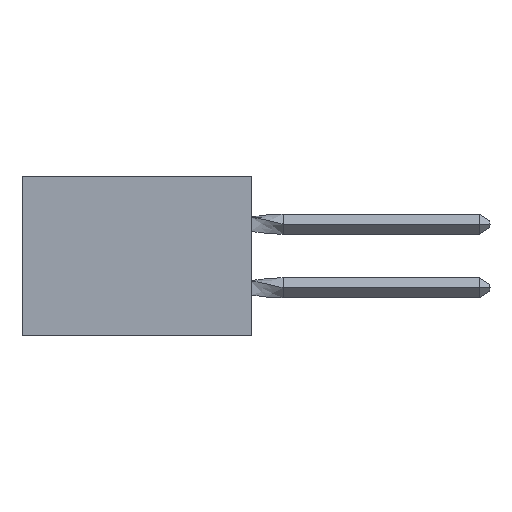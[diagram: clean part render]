
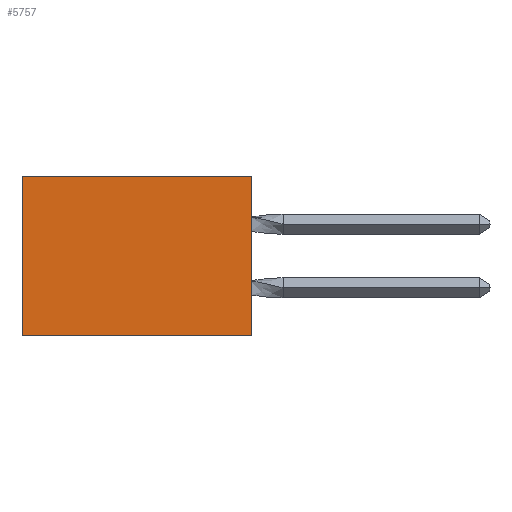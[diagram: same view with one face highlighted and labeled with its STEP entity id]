
A CAD part, left-side view. The second image highlights one B-rep face of the part: STEP entity #5757.
In plain terms, the highlighted planar face has unit normal (-1, 0, 0).
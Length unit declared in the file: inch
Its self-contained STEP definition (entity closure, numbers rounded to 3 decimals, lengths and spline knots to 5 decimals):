
#210 = EDGE_LOOP ( 'NONE', ( #7319, #8463, #7004, #6619 ) ) ;
#682 = VERTEX_POINT ( 'NONE', #9367 ) ;
#1037 = DIRECTION ( 'NONE',  ( 0., 0., -1. ) ) ;
#1528 = CARTESIAN_POINT ( 'NONE',  ( 0.305, 0.72, 0. ) ) ;
#1674 = DIRECTION ( 'NONE',  ( 0., 0., -1. ) ) ;
#1852 = EDGE_CURVE ( 'NONE', #682, #4171, #11782, .T. ) ;
#2416 = EDGE_CURVE ( 'NONE', #11622, #5801, #9221, .T. ) ;
#3059 = DIRECTION ( 'NONE',  ( 0., 1., 0. ) ) ;
#3100 = CARTESIAN_POINT ( 'NONE',  ( 0.305, 0., -0.5 ) ) ;
#3470 = AXIS2_PLACEMENT_3D ( 'NONE', #13197, #12264, #11199 ) ;
#3855 = VECTOR ( 'NONE', #3059, 39.37008 ) ;
#4153 = CARTESIAN_POINT ( 'NONE',  ( 0.305, 0.72, -0.5 ) ) ;
#4171 = VERTEX_POINT ( 'NONE', #1528 ) ;
#4537 = VECTOR ( 'NONE', #1037, 39.37008 ) ;
#5192 = LINE ( 'NONE', #12536, #4537 ) ;
#5757 = ADVANCED_FACE ( 'NONE', ( #7656 ), #6988, .F. ) ;
#5801 = VERTEX_POINT ( 'NONE', #4153 ) ;
#6090 = DIRECTION ( 'NONE',  ( 0., 1., 0. ) ) ;
#6619 = ORIENTED_EDGE ( 'NONE', *, *, #1852, .T. ) ;
#6805 = VECTOR ( 'NONE', #1674, 39.37008 ) ;
#6988 = PLANE ( 'NONE',  #3470 ) ;
#7004 = ORIENTED_EDGE ( 'NONE', *, *, #11348, .F. ) ;
#7319 = ORIENTED_EDGE ( 'NONE', *, *, #13141, .T. ) ;
#7656 = FACE_OUTER_BOUND ( 'NONE', #210, .T. ) ;
#8463 = ORIENTED_EDGE ( 'NONE', *, *, #2416, .F. ) ;
#8894 = CARTESIAN_POINT ( 'NONE',  ( 0.305, 0., -0.5 ) ) ;
#9221 = LINE ( 'NONE', #3100, #9873 ) ;
#9367 = CARTESIAN_POINT ( 'NONE',  ( 0.305, 0., 0. ) ) ;
#9584 = LINE ( 'NONE', #13282, #6805 ) ;
#9873 = VECTOR ( 'NONE', #6090, 39.37008 ) ;
#11199 = DIRECTION ( 'NONE',  ( 0., 0., -1. ) ) ;
#11348 = EDGE_CURVE ( 'NONE', #682, #11622, #5192, .T. ) ;
#11622 = VERTEX_POINT ( 'NONE', #8894 ) ;
#11782 = LINE ( 'NONE', #13550, #3855 ) ;
#12264 = DIRECTION ( 'NONE',  ( 1., 0., 0. ) ) ;
#12536 = CARTESIAN_POINT ( 'NONE',  ( 0.305, 0., -0.5 ) ) ;
#13141 = EDGE_CURVE ( 'NONE', #4171, #5801, #9584, .T. ) ;
#13197 = CARTESIAN_POINT ( 'NONE',  ( 0.305, 0., -0.5 ) ) ;
#13282 = CARTESIAN_POINT ( 'NONE',  ( 0.305, 0.72, -0.5 ) ) ;
#13550 = CARTESIAN_POINT ( 'NONE',  ( 0.305, 0., 0. ) ) ;
